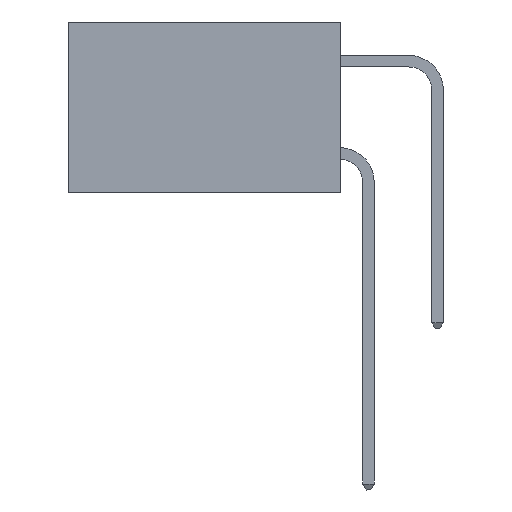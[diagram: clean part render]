
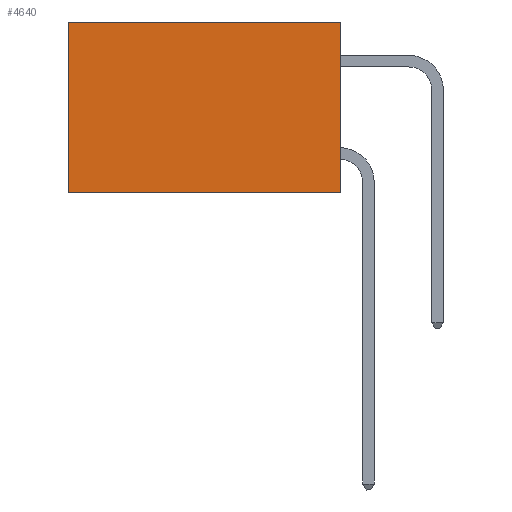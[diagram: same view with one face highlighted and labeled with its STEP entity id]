
A CAD part, left-side view. The second image highlights one B-rep face of the part: STEP entity #4640.
In plain terms, the highlighted planar face has unit normal (-1, 0, 0).
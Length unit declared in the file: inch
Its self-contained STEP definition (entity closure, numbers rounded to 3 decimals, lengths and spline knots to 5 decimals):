
#87 = ORIENTED_EDGE ( 'NONE', *, *, #124, .T. ) ;
#124 = EDGE_CURVE ( 'NONE', #8925, #2846, #7472, .T. ) ;
#914 = AXIS2_PLACEMENT_3D ( 'NONE', #5647, #5639, #5611 ) ;
#979 = DIRECTION ( 'NONE',  ( 0., 1., 0. ) ) ;
#1330 = VERTEX_POINT ( 'NONE', #4562 ) ;
#1344 = DIRECTION ( 'NONE',  ( 0., 0., -1. ) ) ;
#1584 = DIRECTION ( 'NONE',  ( 0., 0., -1. ) ) ;
#1904 = VECTOR ( 'NONE', #3087, 39.37008 ) ;
#2057 = ORIENTED_EDGE ( 'NONE', *, *, #4141, .F. ) ;
#2413 = CARTESIAN_POINT ( 'NONE',  ( 0.277, 0.59, 0. ) ) ;
#2428 = CARTESIAN_POINT ( 'NONE',  ( 0.277, 0.59, -0.37 ) ) ;
#2743 = EDGE_LOOP ( 'NONE', ( #4049, #8251, #2057, #87 ) ) ;
#2818 = CARTESIAN_POINT ( 'NONE',  ( 0.277, 0., 0. ) ) ;
#2846 = VERTEX_POINT ( 'NONE', #2413 ) ;
#3012 = EDGE_CURVE ( 'NONE', #2846, #1330, #6498, .T. ) ;
#3087 = DIRECTION ( 'NONE',  ( 0., 1., 0. ) ) ;
#3284 = CARTESIAN_POINT ( 'NONE',  ( 0.277, 0., -0.37 ) ) ;
#3719 = CARTESIAN_POINT ( 'NONE',  ( 0.277, 0., -0.37 ) ) ;
#4049 = ORIENTED_EDGE ( 'NONE', *, *, #3012, .T. ) ;
#4110 = EDGE_CURVE ( 'NONE', #7055, #1330, #6342, .T. ) ;
#4141 = EDGE_CURVE ( 'NONE', #8925, #7055, #7872, .T. ) ;
#4322 = VECTOR ( 'NONE', #1584, 39.37008 ) ;
#4562 = CARTESIAN_POINT ( 'NONE',  ( 0.277, 0.59, -0.37 ) ) ;
#4640 = ADVANCED_FACE ( 'NONE', ( #6686 ), #6305, .F. ) ;
#5611 = DIRECTION ( 'NONE',  ( 0., 0., -1. ) ) ;
#5639 = DIRECTION ( 'NONE',  ( 1., 0., 0. ) ) ;
#5647 = CARTESIAN_POINT ( 'NONE',  ( 0.277, 0., -0.37 ) ) ;
#5846 = VECTOR ( 'NONE', #1344, 39.37008 ) ;
#6305 = PLANE ( 'NONE',  #914 ) ;
#6342 = LINE ( 'NONE', #3284, #1904 ) ;
#6498 = LINE ( 'NONE', #2428, #4322 ) ;
#6642 = CARTESIAN_POINT ( 'NONE',  ( 0.277, 0., 0. ) ) ;
#6686 = FACE_OUTER_BOUND ( 'NONE', #2743, .T. ) ;
#7055 = VERTEX_POINT ( 'NONE', #7530 ) ;
#7238 = VECTOR ( 'NONE', #979, 39.37008 ) ;
#7472 = LINE ( 'NONE', #6642, #7238 ) ;
#7530 = CARTESIAN_POINT ( 'NONE',  ( 0.277, 0., -0.37 ) ) ;
#7872 = LINE ( 'NONE', #3719, #5846 ) ;
#8251 = ORIENTED_EDGE ( 'NONE', *, *, #4110, .F. ) ;
#8925 = VERTEX_POINT ( 'NONE', #2818 ) ;
